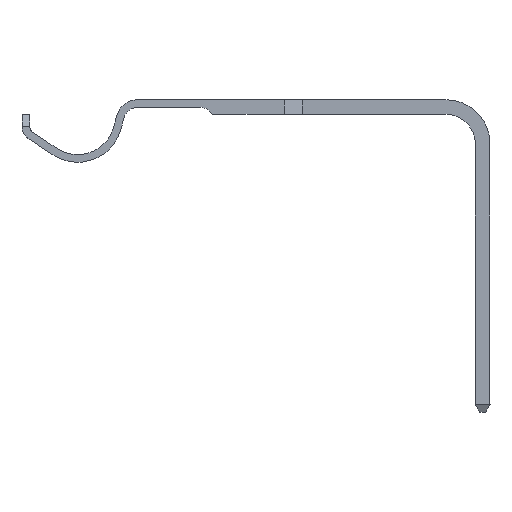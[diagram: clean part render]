
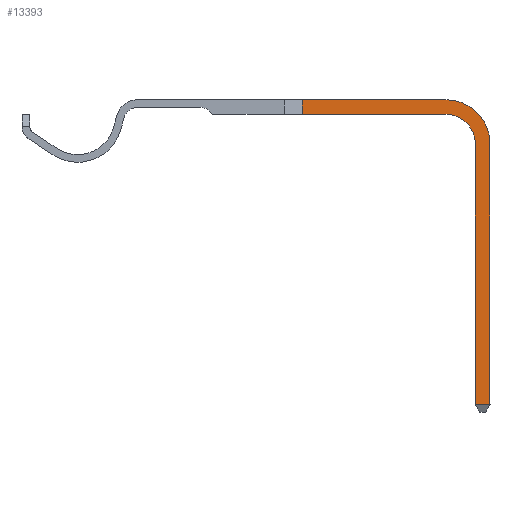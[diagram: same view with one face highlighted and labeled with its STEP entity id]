
A CAD part, left-side view. The second image highlights one B-rep face of the part: STEP entity #13393.
In plain terms, the highlighted face is planar.
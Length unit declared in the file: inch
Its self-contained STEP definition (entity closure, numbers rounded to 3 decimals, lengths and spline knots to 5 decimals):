
#792 = VERTEX_POINT ( 'NONE', #5036 ) ;
#811 = VERTEX_POINT ( 'NONE', #1632 ) ;
#834 = CARTESIAN_POINT ( 'NONE',  ( 0.85571, 0.532, -0.0125 ) ) ;
#980 = EDGE_CURVE ( 'NONE', #8144, #811, #15468, .T. ) ;
#1510 = DIRECTION ( 'NONE',  ( 0., 0., -1. ) ) ;
#1596 = CARTESIAN_POINT ( 'NONE',  ( 0.93071, 0.532, -0.0125 ) ) ;
#1632 = CARTESIAN_POINT ( 'NONE',  ( 0.85571, 0.0125, -0.0125 ) ) ;
#1783 = LINE ( 'NONE', #4791, #9117 ) ;
#1893 = EDGE_CURVE ( 'NONE', #792, #2038, #5926, .T. ) ;
#1916 = CARTESIAN_POINT ( 'NONE',  ( 0.61115, 0.0375, -0.0125 ) ) ;
#2038 = VERTEX_POINT ( 'NONE', #1596 ) ;
#2184 = ORIENTED_EDGE ( 'NONE', *, *, #15562, .T. ) ;
#2229 = CARTESIAN_POINT ( 'NONE',  ( 0.85571, 0.0875, -0.0125 ) ) ;
#2783 = ORIENTED_EDGE ( 'NONE', *, *, #19974, .T. ) ;
#3204 = CARTESIAN_POINT ( 'NONE',  ( 0.61115, 0.0125, -0.0125 ) ) ;
#3484 = ORIENTED_EDGE ( 'NONE', *, *, #14143, .T. ) ;
#3752 = EDGE_LOOP ( 'NONE', ( #17160, #5517, #2184, #13015, #19070, #6357, #3484, #2783 ) ) ;
#3776 = DIRECTION ( 'NONE',  ( 0., 0., 1. ) ) ;
#4386 = EDGE_CURVE ( 'NONE', #811, #9940, #9167, .T. ) ;
#4442 = CARTESIAN_POINT ( 'NONE',  ( 0.58021, 0.0375, -0.0125 ) ) ;
#4460 = DIRECTION ( 'NONE',  ( 0., 0., 1. ) ) ;
#4478 = DIRECTION ( 'NONE',  ( -1., 0., 0. ) ) ;
#4791 = CARTESIAN_POINT ( 'NONE',  ( 0.61115, 0.0875, -0.0125 ) ) ;
#5009 = FACE_OUTER_BOUND ( 'NONE', #3752, .T. ) ;
#5036 = CARTESIAN_POINT ( 'NONE',  ( 0.90571, 0.532, -0.0125 ) ) ;
#5517 = ORIENTED_EDGE ( 'NONE', *, *, #1893, .T. ) ;
#5624 = CIRCLE ( 'NONE', #7140, 0.05 ) ;
#5813 = EDGE_CURVE ( 'NONE', #10278, #792, #14593, .T. ) ;
#5926 = LINE ( 'NONE', #834, #18180 ) ;
#5992 = DIRECTION ( 'NONE',  ( 1., 0., 0. ) ) ;
#6240 = DIRECTION ( 'NONE',  ( 1., 0., 0. ) ) ;
#6357 = ORIENTED_EDGE ( 'NONE', *, *, #15533, .T. ) ;
#6924 = AXIS2_PLACEMENT_3D ( 'NONE', #2229, #3776, #14855 ) ;
#6928 = LINE ( 'NONE', #4442, #19188 ) ;
#7140 = AXIS2_PLACEMENT_3D ( 'NONE', #13953, #4460, #15581 ) ;
#7518 = CARTESIAN_POINT ( 'NONE',  ( 0.90571, 0.0875, -0.0125 ) ) ;
#7965 = DIRECTION ( 'NONE',  ( 0., -1., 0. ) ) ;
#8144 = VERTEX_POINT ( 'NONE', #14394 ) ;
#8184 = VERTEX_POINT ( 'NONE', #1916 ) ;
#8348 = CARTESIAN_POINT ( 'NONE',  ( 0.85571, 0.0875, -0.0125 ) ) ;
#9117 = VECTOR ( 'NONE', #12691, 39.37008 ) ;
#9167 = LINE ( 'NONE', #16009, #13909 ) ;
#9586 = CARTESIAN_POINT ( 'NONE',  ( 0.93071, 0.0875, -0.0125 ) ) ;
#9940 = VERTEX_POINT ( 'NONE', #3204 ) ;
#10278 = VERTEX_POINT ( 'NONE', #16675 ) ;
#11641 = PLANE ( 'NONE',  #6924 ) ;
#12691 = DIRECTION ( 'NONE',  ( 0., 1., 0. ) ) ;
#12847 = VECTOR ( 'NONE', #7965, 39.37008 ) ;
#12869 = CARTESIAN_POINT ( 'NONE',  ( 0.85571, 0.0375, -0.0125 ) ) ;
#13015 = ORIENTED_EDGE ( 'NONE', *, *, #980, .T. ) ;
#13365 = VERTEX_POINT ( 'NONE', #12869 ) ;
#13393 = ADVANCED_FACE ( 'NONE', ( #5009 ), #11641, .F. ) ;
#13909 = VECTOR ( 'NONE', #4478, 39.37008 ) ;
#13953 = CARTESIAN_POINT ( 'NONE',  ( 0.85571, 0.0875, -0.0125 ) ) ;
#14088 = VECTOR ( 'NONE', #20279, 39.37008 ) ;
#14143 = EDGE_CURVE ( 'NONE', #8184, #13365, #6928, .T. ) ;
#14394 = CARTESIAN_POINT ( 'NONE',  ( 0.93071, 0.0875, -0.0125 ) ) ;
#14593 = LINE ( 'NONE', #7518, #14088 ) ;
#14855 = DIRECTION ( 'NONE',  ( 1., 0., 0. ) ) ;
#15468 = CIRCLE ( 'NONE', #20274, 0.075 ) ;
#15533 = EDGE_CURVE ( 'NONE', #9940, #8184, #1783, .T. ) ;
#15562 = EDGE_CURVE ( 'NONE', #2038, #8144, #17099, .T. ) ;
#15581 = DIRECTION ( 'NONE',  ( 1., 0., 0. ) ) ;
#16009 = CARTESIAN_POINT ( 'NONE',  ( 0.58021, 0.0125, -0.0125 ) ) ;
#16675 = CARTESIAN_POINT ( 'NONE',  ( 0.90571, 0.0875, -0.0125 ) ) ;
#17099 = LINE ( 'NONE', #9586, #12847 ) ;
#17160 = ORIENTED_EDGE ( 'NONE', *, *, #5813, .T. ) ;
#18180 = VECTOR ( 'NONE', #20218, 39.37008 ) ;
#19070 = ORIENTED_EDGE ( 'NONE', *, *, #4386, .T. ) ;
#19188 = VECTOR ( 'NONE', #5992, 39.37008 ) ;
#19974 = EDGE_CURVE ( 'NONE', #13365, #10278, #5624, .T. ) ;
#20218 = DIRECTION ( 'NONE',  ( 1., 0., 0. ) ) ;
#20274 = AXIS2_PLACEMENT_3D ( 'NONE', #8348, #1510, #6240 ) ;
#20279 = DIRECTION ( 'NONE',  ( 0., 1., 0. ) ) ;
